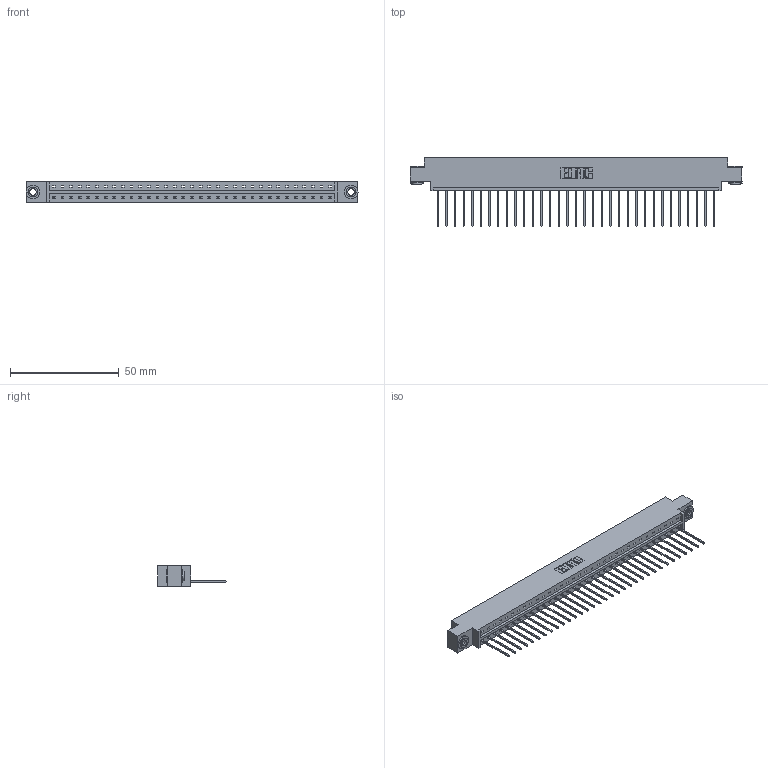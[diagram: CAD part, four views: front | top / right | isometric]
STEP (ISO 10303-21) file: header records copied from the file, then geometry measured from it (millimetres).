
FILE_DESCRIPTION (( 'STEP AP203' ), '1' );
FILE_NAME ('333-033-542-603.STEP', '2018-08-02T21:22:19', ( '' ), ( '' ), 'SwSTEP 2.0', 'SolidWorks 2016', '' );
FILE_SCHEMA (( 'CONFIG_CONTROL_DESIGN' ));
Length unit declared in the file: inch
Products named in the file (4): 345-250-002_345-250-002-102; 333-033-542-603; 333 Part_Offset - .156 Dia - TH; 345-292-001_345-293-142
Assembly tree (36 placements, depth 2):
  333-033-542-603
    333 Part_Offset - .156 Dia - TH
    345-292-001_345-293-142  x33
    345-250-002_345-250-002-102  x2
Bounding box: 152.3 x 31.63 x 9.4 mm (x, y, z)
Volume: 15113.1 mm3; surface area: 17202.3 mm2
Topology: 36 solids, 36 shells, 2070 faces, 6207 edges, 4090 vertices
Faces by surface type: plane 1470, cylinder 592, cone 8
Entity records: 22138 total; most frequent: CARTESIAN_POINT 3800, ORIENTED_EDGE 3762, DIRECTION 3257, EDGE_CURVE 1881, VECTOR 1729, LINE 1729, VERTEX_POINT 1250, AXIS2_PLACEMENT_3D 764
